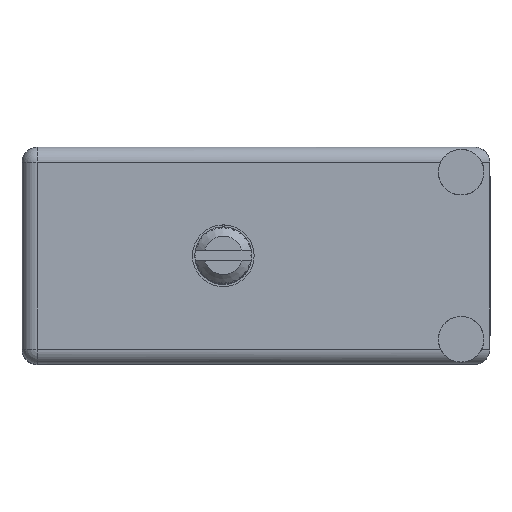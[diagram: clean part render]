
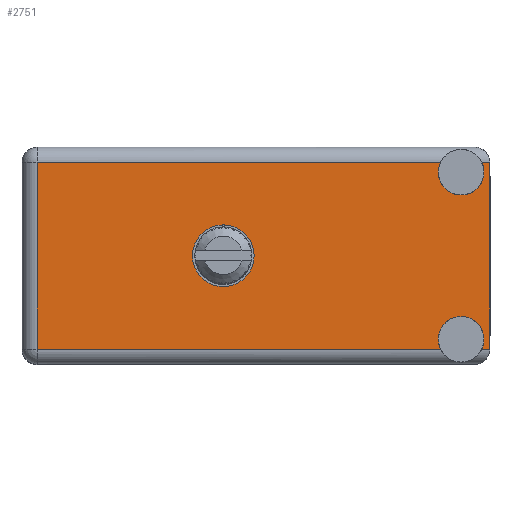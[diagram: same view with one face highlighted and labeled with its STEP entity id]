
A CAD part, top view. The second image highlights one B-rep face of the part: STEP entity #2751.
In plain terms, the highlighted face is planar.
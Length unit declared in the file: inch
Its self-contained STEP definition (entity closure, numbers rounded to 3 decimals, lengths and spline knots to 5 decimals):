
#2751 = ADVANCED_FACE ( 'NONE', ( #100697, #186346 ), #134937, .T. ) ;
#4870 = VECTOR ( 'NONE', #97651, 39.37008 ) ;
#5452 = EDGE_CURVE ( 'NONE', #13245, #111380, #23786, .T. ) ;
#6474 = CARTESIAN_POINT ( 'NONE',  ( -0.6625, 0.806, -0.3575 ) ) ;
#7755 = LINE ( 'NONE', #41907, #16779 ) ;
#10025 = CARTESIAN_POINT ( 'NONE',  ( 0.8765, 0.806, -0.3075 ) ) ;
#11072 = DIRECTION ( 'NONE',  ( -1., 0., 0. ) ) ;
#11583 = DIRECTION ( 'NONE',  ( 0., 0., 1. ) ) ;
#12627 = EDGE_LOOP ( 'NONE', ( #158787, #72984, #66937, #112085, #60125, #86274, #99042, #53540, #56084, #28429 ) ) ;
#12973 = VERTEX_POINT ( 'NONE', #33695 ) ;
#13245 = VERTEX_POINT ( 'NONE', #35349 ) ;
#15111 = AXIS2_PLACEMENT_3D ( 'NONE', #57424, #42926, #113483 ) ;
#16779 = VECTOR ( 'NONE', #156007, 39.37008 ) ;
#18986 = EDGE_CURVE ( 'NONE', #46840, #150316, #109131, .T. ) ;
#20098 = CARTESIAN_POINT ( 'NONE',  ( 0.8765, 0.806, 0.3575 ) ) ;
#21341 = DIRECTION ( 'NONE',  ( 0., 0., 1. ) ) ;
#21591 = DIRECTION ( 'NONE',  ( 0., 1., 0. ) ) ;
#21877 = EDGE_CURVE ( 'NONE', #12973, #157129, #106192, .T. ) ;
#23748 = CIRCLE ( 'NONE', #114888, 0.075 ) ;
#23786 = CIRCLE ( 'NONE', #99643, 0.1015 ) ;
#25807 = CARTESIAN_POINT ( 'NONE',  ( 0.85009, 0.806, -0.3075 ) ) ;
#27835 = DIRECTION ( 'NONE',  ( 0., 1., 0. ) ) ;
#27956 = CARTESIAN_POINT ( 'NONE',  ( 0.71491, 0.806, -0.3075 ) ) ;
#28141 = CIRCLE ( 'NONE', #125121, 0.1015 ) ;
#28429 = ORIENTED_EDGE ( 'NONE', *, *, #128002, .T. ) ;
#30479 = VERTEX_POINT ( 'NONE', #117323 ) ;
#33695 = CARTESIAN_POINT ( 'NONE',  ( 0.85009, 0.806, 0.3075 ) ) ;
#35349 = CARTESIAN_POINT ( 'NONE',  ( 0., 0.806, -0.1015 ) ) ;
#36991 = EDGE_CURVE ( 'NONE', #46840, #157129, #90308, .T. ) ;
#37342 = VERTEX_POINT ( 'NONE', #181014 ) ;
#38463 = CARTESIAN_POINT ( 'NONE',  ( 0.8765, 0.806, 0.3075 ) ) ;
#39929 = DIRECTION ( 'NONE',  ( 0., 0., 1. ) ) ;
#41907 = CARTESIAN_POINT ( 'NONE',  ( 0.8765, 0.806, 0.3075 ) ) ;
#42315 = DIRECTION ( 'NONE',  ( 0., 1., 0. ) ) ;
#42926 = DIRECTION ( 'NONE',  ( 0., 1., 0. ) ) ;
#46840 = VERTEX_POINT ( 'NONE', #10025 ) ;
#47128 = DIRECTION ( 'NONE',  ( 0., 0., 1. ) ) ;
#50317 = EDGE_LOOP ( 'NONE', ( #132886, #177283 ) ) ;
#53207 = CARTESIAN_POINT ( 'NONE',  ( -0.6125, 0.806, -0.3075 ) ) ;
#53540 = ORIENTED_EDGE ( 'NONE', *, *, #175121, .F. ) ;
#54078 = AXIS2_PLACEMENT_3D ( 'NONE', #70086, #42315, #11583 ) ;
#56084 = ORIENTED_EDGE ( 'NONE', *, *, #121609, .T. ) ;
#56509 = VECTOR ( 'NONE', #21341, 39.37008 ) ;
#57424 = CARTESIAN_POINT ( 'NONE',  ( 0.7825, 0.806, 0.275 ) ) ;
#60125 = ORIENTED_EDGE ( 'NONE', *, *, #36991, .F. ) ;
#66937 = ORIENTED_EDGE ( 'NONE', *, *, #69238, .F. ) ;
#69238 = EDGE_CURVE ( 'NONE', #12973, #85939, #154744, .T. ) ;
#69881 = CIRCLE ( 'NONE', #15111, 0.075 ) ;
#70086 = CARTESIAN_POINT ( 'NONE',  ( 0.7825, 0.806, -0.275 ) ) ;
#71181 = DIRECTION ( 'NONE',  ( 0., 0., 1. ) ) ;
#71324 = CARTESIAN_POINT ( 'NONE',  ( 0., 0.806, 0. ) ) ;
#72984 = ORIENTED_EDGE ( 'NONE', *, *, #100976, .F. ) ;
#74314 = CARTESIAN_POINT ( 'NONE',  ( 0., 0.806, 0. ) ) ;
#74927 = DIRECTION ( 'NONE',  ( 0., 1., 0. ) ) ;
#81449 = EDGE_CURVE ( 'NONE', #111380, #13245, #28141, .T. ) ;
#84564 = AXIS2_PLACEMENT_3D ( 'NONE', #157457, #155603, #71181 ) ;
#84646 = CARTESIAN_POINT ( 'NONE',  ( 0.7825, 0.806, -0.275 ) ) ;
#84975 = CARTESIAN_POINT ( 'NONE',  ( 0., 0.806, 0.1015 ) ) ;
#85939 = VERTEX_POINT ( 'NONE', #151730 ) ;
#86274 = ORIENTED_EDGE ( 'NONE', *, *, #18986, .T. ) ;
#87076 = DIRECTION ( 'NONE',  ( -1., 0., 0. ) ) ;
#88306 = VECTOR ( 'NONE', #153340, 39.37008 ) ;
#90308 = LINE ( 'NONE', #20098, #56509 ) ;
#93863 = CARTESIAN_POINT ( 'NONE',  ( 0.71491, 0.806, 0.3075 ) ) ;
#97651 = DIRECTION ( 'NONE',  ( 1., 0., 0. ) ) ;
#99010 = DIRECTION ( 'NONE',  ( 0., 0., 1. ) ) ;
#99042 = ORIENTED_EDGE ( 'NONE', *, *, #146508, .F. ) ;
#99643 = AXIS2_PLACEMENT_3D ( 'NONE', #71324, #27835, #99010 ) ;
#100697 = FACE_BOUND ( 'NONE', #50317, .T. ) ;
#100976 = EDGE_CURVE ( 'NONE', #85939, #177717, #69881, .T. ) ;
#106192 = LINE ( 'NONE', #38463, #4870 ) ;
#109131 = LINE ( 'NONE', #128651, #138410 ) ;
#111380 = VERTEX_POINT ( 'NONE', #84975 ) ;
#112085 = ORIENTED_EDGE ( 'NONE', *, *, #21877, .T. ) ;
#112938 = DIRECTION ( 'NONE',  ( 0., 1., 0. ) ) ;
#113483 = DIRECTION ( 'NONE',  ( 0., 0., 1. ) ) ;
#114154 = CIRCLE ( 'NONE', #54078, 0.075 ) ;
#114888 = AXIS2_PLACEMENT_3D ( 'NONE', #84646, #112938, #39929 ) ;
#117323 = CARTESIAN_POINT ( 'NONE',  ( 0.7825, 0.806, -0.2 ) ) ;
#118839 = VECTOR ( 'NONE', #11072, 39.37008 ) ;
#121609 = EDGE_CURVE ( 'NONE', #146664, #146641, #159368, .T. ) ;
#122325 = DIRECTION ( 'NONE',  ( -1., 0., 0. ) ) ;
#125018 = CARTESIAN_POINT ( 'NONE',  ( -0.6625, 0.806, -0.3075 ) ) ;
#125121 = AXIS2_PLACEMENT_3D ( 'NONE', #74314, #74927, #47128 ) ;
#125889 = AXIS2_PLACEMENT_3D ( 'NONE', #6474, #21591, #122325 ) ;
#128002 = EDGE_CURVE ( 'NONE', #146641, #37342, #131113, .T. ) ;
#128651 = CARTESIAN_POINT ( 'NONE',  ( -0.6625, 0.806, -0.3075 ) ) ;
#131113 = LINE ( 'NONE', #138854, #88306 ) ;
#132886 = ORIENTED_EDGE ( 'NONE', *, *, #81449, .F. ) ;
#133484 = CARTESIAN_POINT ( 'NONE',  ( 0.8765, 0.806, 0.3075 ) ) ;
#134937 = PLANE ( 'NONE',  #125889 ) ;
#138410 = VECTOR ( 'NONE', #87076, 39.37008 ) ;
#138854 = CARTESIAN_POINT ( 'NONE',  ( -0.6125, 0.806, -0.3575 ) ) ;
#146508 = EDGE_CURVE ( 'NONE', #30479, #150316, #23748, .T. ) ;
#146641 = VERTEX_POINT ( 'NONE', #53207 ) ;
#146664 = VERTEX_POINT ( 'NONE', #27956 ) ;
#150316 = VERTEX_POINT ( 'NONE', #25807 ) ;
#151730 = CARTESIAN_POINT ( 'NONE',  ( 0.7825, 0.806, 0.2 ) ) ;
#153340 = DIRECTION ( 'NONE',  ( 0., 0., 1. ) ) ;
#153943 = EDGE_CURVE ( 'NONE', #37342, #177717, #7755, .T. ) ;
#154744 = CIRCLE ( 'NONE', #84564, 0.075 ) ;
#155603 = DIRECTION ( 'NONE',  ( 0., 1., 0. ) ) ;
#156007 = DIRECTION ( 'NONE',  ( 1., 0., 0. ) ) ;
#157129 = VERTEX_POINT ( 'NONE', #133484 ) ;
#157457 = CARTESIAN_POINT ( 'NONE',  ( 0.7825, 0.806, 0.275 ) ) ;
#158787 = ORIENTED_EDGE ( 'NONE', *, *, #153943, .T. ) ;
#159368 = LINE ( 'NONE', #125018, #118839 ) ;
#175121 = EDGE_CURVE ( 'NONE', #146664, #30479, #114154, .T. ) ;
#177283 = ORIENTED_EDGE ( 'NONE', *, *, #5452, .F. ) ;
#177717 = VERTEX_POINT ( 'NONE', #93863 ) ;
#181014 = CARTESIAN_POINT ( 'NONE',  ( -0.6125, 0.806, 0.3075 ) ) ;
#186346 = FACE_OUTER_BOUND ( 'NONE', #12627, .T. ) ;
